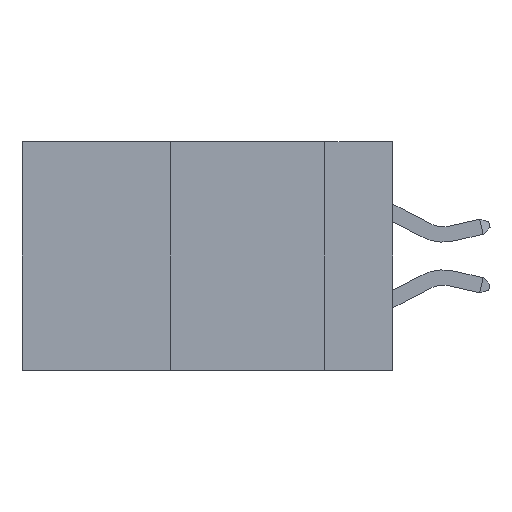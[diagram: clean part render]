
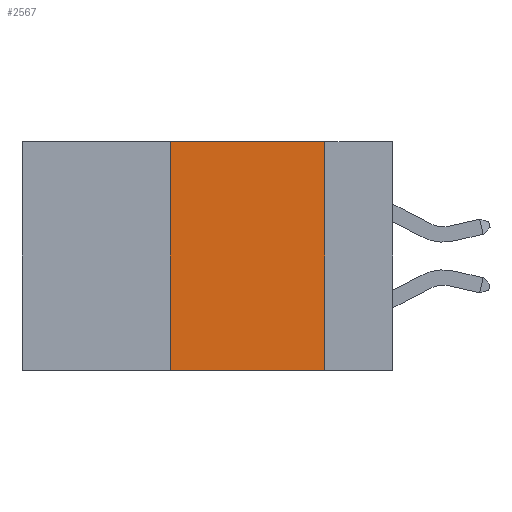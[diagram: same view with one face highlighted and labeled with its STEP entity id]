
A CAD part, left-side view. The second image highlights one B-rep face of the part: STEP entity #2567.
In plain terms, the highlighted planar face has unit normal (-1, 0, 0).
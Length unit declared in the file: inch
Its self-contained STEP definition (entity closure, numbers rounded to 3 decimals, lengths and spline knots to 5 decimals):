
#2149 = CARTESIAN_POINT ( 'NONE',  ( 0., 0.6, 0. ) ) ;
#2567 = ADVANCED_FACE ( 'NONE', ( #19472 ), #6553, .F. ) ;
#2965 = CARTESIAN_POINT ( 'NONE',  ( 0., 0.11, -0.37 ) ) ;
#3696 = CARTESIAN_POINT ( 'NONE',  ( 0., 0.11, 0. ) ) ;
#3781 = CARTESIAN_POINT ( 'NONE',  ( 0., 0.6, -0.37 ) ) ;
#4907 = VERTEX_POINT ( 'NONE', #8832 ) ;
#5042 = DIRECTION ( 'NONE',  ( 0., -1., 0. ) ) ;
#5696 = CARTESIAN_POINT ( 'NONE',  ( 0., 0.6, 0. ) ) ;
#6553 = PLANE ( 'NONE',  #12556 ) ;
#6689 = VECTOR ( 'NONE', #10664, 39.37008 ) ;
#7168 = LINE ( 'NONE', #5696, #6689 ) ;
#7475 = EDGE_CURVE ( 'NONE', #8786, #14324, #10218, .T. ) ;
#8786 = VERTEX_POINT ( 'NONE', #15306 ) ;
#8832 = CARTESIAN_POINT ( 'NONE',  ( 0., 0.36, 0. ) ) ;
#9052 = VERTEX_POINT ( 'NONE', #3696 ) ;
#9727 = ORIENTED_EDGE ( 'NONE', *, *, #19580, .F. ) ;
#9759 = LINE ( 'NONE', #12909, #10962 ) ;
#10218 = LINE ( 'NONE', #3781, #17608 ) ;
#10311 = DIRECTION ( 'NONE',  ( 0., 0., 1. ) ) ;
#10572 = EDGE_LOOP ( 'NONE', ( #13966, #9727, #14251, #20741 ) ) ;
#10664 = DIRECTION ( 'NONE',  ( 0., -1., 0. ) ) ;
#10962 = VECTOR ( 'NONE', #19191, 39.37008 ) ;
#11637 = EDGE_CURVE ( 'NONE', #9052, #14324, #9759, .T. ) ;
#12556 = AXIS2_PLACEMENT_3D ( 'NONE', #2149, #13192, #17903 ) ;
#12909 = CARTESIAN_POINT ( 'NONE',  ( 0., 0.11, 0. ) ) ;
#13192 = DIRECTION ( 'NONE',  ( 1., 0., 0. ) ) ;
#13966 = ORIENTED_EDGE ( 'NONE', *, *, #11637, .F. ) ;
#14251 = ORIENTED_EDGE ( 'NONE', *, *, #18602, .F. ) ;
#14324 = VERTEX_POINT ( 'NONE', #2965 ) ;
#15306 = CARTESIAN_POINT ( 'NONE',  ( 0., 0.36, -0.37 ) ) ;
#17006 = LINE ( 'NONE', #18685, #20124 ) ;
#17608 = VECTOR ( 'NONE', #5042, 39.37008 ) ;
#17903 = DIRECTION ( 'NONE',  ( 0., 0., -1. ) ) ;
#18602 = EDGE_CURVE ( 'NONE', #8786, #4907, #17006, .T. ) ;
#18685 = CARTESIAN_POINT ( 'NONE',  ( 0., 0.36, 0. ) ) ;
#19191 = DIRECTION ( 'NONE',  ( 0., 0., -1. ) ) ;
#19472 = FACE_OUTER_BOUND ( 'NONE', #10572, .T. ) ;
#19580 = EDGE_CURVE ( 'NONE', #4907, #9052, #7168, .T. ) ;
#20124 = VECTOR ( 'NONE', #10311, 39.37008 ) ;
#20741 = ORIENTED_EDGE ( 'NONE', *, *, #7475, .T. ) ;
